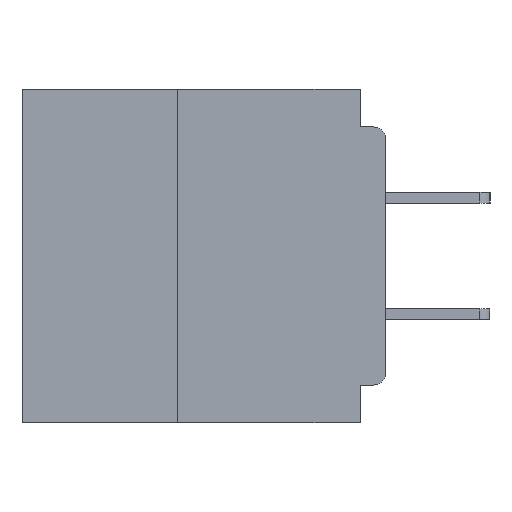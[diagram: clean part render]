
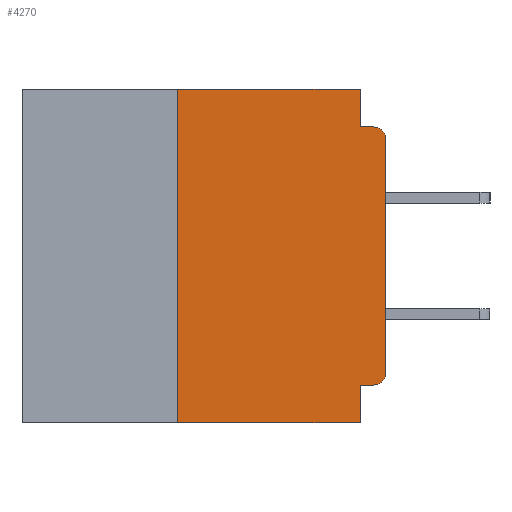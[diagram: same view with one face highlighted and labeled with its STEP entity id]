
A CAD part, left-side view. The second image highlights one B-rep face of the part: STEP entity #4270.
In plain terms, the highlighted planar face has unit normal (-1, 0, 0).
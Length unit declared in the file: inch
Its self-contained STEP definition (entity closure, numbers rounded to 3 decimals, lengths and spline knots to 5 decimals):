
#846 = DIRECTION ( 'NONE',  ( 0., 0., -1. ) ) ;
#855 = DIRECTION ( 'NONE',  ( 1., 0., 0. ) ) ;
#921 = VERTEX_POINT ( 'NONE', #10697 ) ;
#1219 = PLANE ( 'NONE',  #20661 ) ;
#1275 = CARTESIAN_POINT ( 'NONE',  ( 0., 0.437, 0. ) ) ;
#3424 = CARTESIAN_POINT ( 'NONE',  ( 0., 0.015, -0.06 ) ) ;
#3836 = CARTESIAN_POINT ( 'NONE',  ( 0., 0.25, -0.4 ) ) ;
#4270 = ADVANCED_FACE ( 'NONE', ( #44872 ), #1219, .F. ) ;
#4450 = ORIENTED_EDGE ( 'NONE', *, *, #26271, .T. ) ;
#4482 = LINE ( 'NONE', #10682, #46815 ) ;
#6127 = ORIENTED_EDGE ( 'NONE', *, *, #14483, .T. ) ;
#6626 = ORIENTED_EDGE ( 'NONE', *, *, #13809, .F. ) ;
#7147 = DIRECTION ( 'NONE',  ( 0., -1., 0. ) ) ;
#7549 = DIRECTION ( 'NONE',  ( 0., 0., -1. ) ) ;
#7665 = CARTESIAN_POINT ( 'NONE',  ( 0., 0.015, -0.045 ) ) ;
#8229 = EDGE_CURVE ( 'NONE', #12096, #13089, #41502, .T. ) ;
#8310 = CIRCLE ( 'NONE', #41025, 0.015 ) ;
#8793 = ORIENTED_EDGE ( 'NONE', *, *, #8229, .F. ) ;
#10346 = VERTEX_POINT ( 'NONE', #10773 ) ;
#10579 = VECTOR ( 'NONE', #22118, 39.37008 ) ;
#10682 = CARTESIAN_POINT ( 'NONE',  ( 0., 0.25, -0.4 ) ) ;
#10697 = CARTESIAN_POINT ( 'NONE',  ( 0., 0.031, -0.045 ) ) ;
#10773 = CARTESIAN_POINT ( 'NONE',  ( 0., 0.031, 0. ) ) ;
#10852 = DIRECTION ( 'NONE',  ( -1., 0., 0. ) ) ;
#11093 = ORIENTED_EDGE ( 'NONE', *, *, #30341, .T. ) ;
#11340 = ORIENTED_EDGE ( 'NONE', *, *, #33051, .F. ) ;
#11482 = VECTOR ( 'NONE', #45995, 39.37008 ) ;
#12096 = VERTEX_POINT ( 'NONE', #17583 ) ;
#12560 = VERTEX_POINT ( 'NONE', #41913 ) ;
#12742 = LINE ( 'NONE', #17297, #11482 ) ;
#13089 = VERTEX_POINT ( 'NONE', #34783 ) ;
#13809 = EDGE_CURVE ( 'NONE', #34633, #10346, #25474, .T. ) ;
#13947 = VECTOR ( 'NONE', #17570, 39.37008 ) ;
#14365 = CARTESIAN_POINT ( 'NONE',  ( 0., 0., -0.355 ) ) ;
#14483 = EDGE_CURVE ( 'NONE', #12560, #16747, #26026, .T. ) ;
#14688 = DIRECTION ( 'NONE',  ( 0., 0., -1. ) ) ;
#16747 = VERTEX_POINT ( 'NONE', #7665 ) ;
#17297 = CARTESIAN_POINT ( 'NONE',  ( 0., 0., 0. ) ) ;
#17570 = DIRECTION ( 'NONE',  ( 0., 0., -1. ) ) ;
#17583 = CARTESIAN_POINT ( 'NONE',  ( 0., 0.031, -0.355 ) ) ;
#17943 = CARTESIAN_POINT ( 'NONE',  ( 0., 0., -0.045 ) ) ;
#19568 = VECTOR ( 'NONE', #7147, 39.37008 ) ;
#20524 = VERTEX_POINT ( 'NONE', #3836 ) ;
#20661 = AXIS2_PLACEMENT_3D ( 'NONE', #1275, #855, #846 ) ;
#20874 = LINE ( 'NONE', #51856, #19568 ) ;
#22118 = DIRECTION ( 'NONE',  ( 0., -1., 0. ) ) ;
#22441 = CARTESIAN_POINT ( 'NONE',  ( 0., 0., -0.34 ) ) ;
#25474 = LINE ( 'NONE', #51756, #35036 ) ;
#25798 = VERTEX_POINT ( 'NONE', #22441 ) ;
#26026 = CIRCLE ( 'NONE', #29584, 0.015 ) ;
#26233 = LINE ( 'NONE', #46258, #13947 ) ;
#26271 = EDGE_CURVE ( 'NONE', #25798, #12560, #12742, .T. ) ;
#26646 = ORIENTED_EDGE ( 'NONE', *, *, #49378, .F. ) ;
#29584 = AXIS2_PLACEMENT_3D ( 'NONE', #3424, #32240, #7549 ) ;
#30097 = EDGE_CURVE ( 'NONE', #921, #16747, #32514, .T. ) ;
#30341 = EDGE_CURVE ( 'NONE', #20524, #13089, #20874, .T. ) ;
#30743 = VECTOR ( 'NONE', #14688, 39.37008 ) ;
#30849 = DIRECTION ( 'NONE',  ( 0., 1., 0. ) ) ;
#32240 = DIRECTION ( 'NONE',  ( -1., 0., 0. ) ) ;
#32514 = LINE ( 'NONE', #17943, #10579 ) ;
#33051 = EDGE_CURVE ( 'NONE', #20524, #34633, #4482, .T. ) ;
#34599 = ORIENTED_EDGE ( 'NONE', *, *, #30097, .F. ) ;
#34633 = VERTEX_POINT ( 'NONE', #38516 ) ;
#34739 = VERTEX_POINT ( 'NONE', #35294 ) ;
#34783 = CARTESIAN_POINT ( 'NONE',  ( 0., 0.031, -0.4 ) ) ;
#35036 = VECTOR ( 'NONE', #39690, 39.37008 ) ;
#35193 = ORIENTED_EDGE ( 'NONE', *, *, #48469, .T. ) ;
#35294 = CARTESIAN_POINT ( 'NONE',  ( 0., 0.015, -0.355 ) ) ;
#35437 = CARTESIAN_POINT ( 'NONE',  ( 0., 0.015, -0.34 ) ) ;
#37858 = ORIENTED_EDGE ( 'NONE', *, *, #47464, .F. ) ;
#38516 = CARTESIAN_POINT ( 'NONE',  ( 0., 0.25, 0. ) ) ;
#38878 = LINE ( 'NONE', #14365, #48460 ) ;
#39272 = CARTESIAN_POINT ( 'NONE',  ( 0., 0.031, -0.4 ) ) ;
#39372 = DIRECTION ( 'NONE',  ( 0., 0., 1. ) ) ;
#39533 = DIRECTION ( 'NONE',  ( 0., 0., -1. ) ) ;
#39690 = DIRECTION ( 'NONE',  ( 0., -1., 0. ) ) ;
#41025 = AXIS2_PLACEMENT_3D ( 'NONE', #35437, #10852, #39533 ) ;
#41502 = LINE ( 'NONE', #39272, #30743 ) ;
#41913 = CARTESIAN_POINT ( 'NONE',  ( 0., 0., -0.06 ) ) ;
#44766 = EDGE_LOOP ( 'NONE', ( #4450, #6127, #34599, #26646, #6626, #11340, #11093, #8793, #37858, #35193 ) ) ;
#44872 = FACE_OUTER_BOUND ( 'NONE', #44766, .T. ) ;
#45995 = DIRECTION ( 'NONE',  ( 0., 0., 1. ) ) ;
#46258 = CARTESIAN_POINT ( 'NONE',  ( 0., 0.031, 0. ) ) ;
#46815 = VECTOR ( 'NONE', #39372, 39.37008 ) ;
#47464 = EDGE_CURVE ( 'NONE', #34739, #12096, #38878, .T. ) ;
#48460 = VECTOR ( 'NONE', #30849, 39.37008 ) ;
#48469 = EDGE_CURVE ( 'NONE', #34739, #25798, #8310, .T. ) ;
#49378 = EDGE_CURVE ( 'NONE', #10346, #921, #26233, .T. ) ;
#51756 = CARTESIAN_POINT ( 'NONE',  ( 0., 0.437, 0. ) ) ;
#51856 = CARTESIAN_POINT ( 'NONE',  ( 0., 0.437, -0.4 ) ) ;
